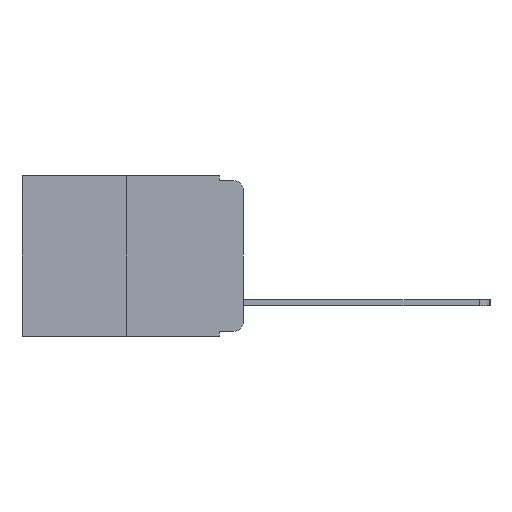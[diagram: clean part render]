
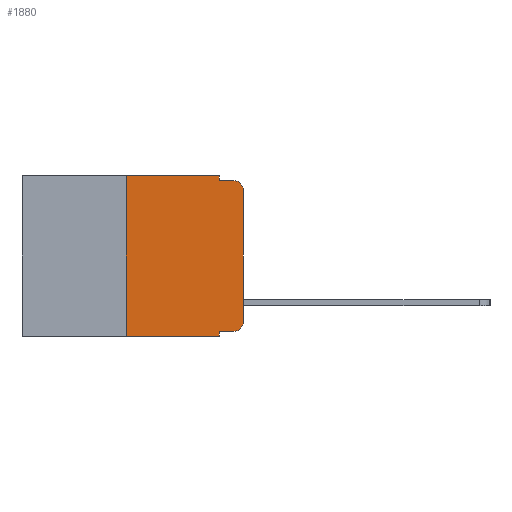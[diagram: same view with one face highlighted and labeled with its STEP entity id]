
A CAD part, left-side view. The second image highlights one B-rep face of the part: STEP entity #1880.
In plain terms, the highlighted planar face has unit normal (-1, 0, 0).
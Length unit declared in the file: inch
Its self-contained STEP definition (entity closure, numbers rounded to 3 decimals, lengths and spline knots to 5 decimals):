
#370 = LINE ( 'NONE', #4355, #4647 ) ;
#617 = EDGE_CURVE ( 'NONE', #16343, #2538, #10913, .T. ) ;
#1018 = LINE ( 'NONE', #10166, #6738 ) ;
#1031 = AXIS2_PLACEMENT_3D ( 'NONE', #2403, #11668, #3817 ) ;
#1208 = ORIENTED_EDGE ( 'NONE', *, *, #4333, .T. ) ;
#1236 = CIRCLE ( 'NONE', #12113, 0.02 ) ;
#1523 = ORIENTED_EDGE ( 'NONE', *, *, #617, .F. ) ;
#1568 = VERTEX_POINT ( 'NONE', #9383 ) ;
#1818 = VECTOR ( 'NONE', #5130, 39.37008 ) ;
#1880 = ADVANCED_FACE ( 'NONE', ( #2723 ), #7766, .F. ) ;
#2147 = VECTOR ( 'NONE', #4517, 39.37008 ) ;
#2393 = EDGE_CURVE ( 'NONE', #2538, #14943, #10297, .T. ) ;
#2403 = CARTESIAN_POINT ( 'NONE',  ( 0., 0.02, -0.03 ) ) ;
#2442 = VERTEX_POINT ( 'NONE', #16416 ) ;
#2538 = VERTEX_POINT ( 'NONE', #14724 ) ;
#2723 = FACE_OUTER_BOUND ( 'NONE', #16510, .T. ) ;
#2979 = VECTOR ( 'NONE', #11274, 39.37008 ) ;
#3442 = VECTOR ( 'NONE', #6699, 39.37008 ) ;
#3659 = DIRECTION ( 'NONE',  ( 0., -1., 0. ) ) ;
#3817 = DIRECTION ( 'NONE',  ( 0., 0., -1. ) ) ;
#4295 = EDGE_CURVE ( 'NONE', #6112, #16343, #1018, .T. ) ;
#4328 = EDGE_CURVE ( 'NONE', #10841, #12008, #16121, .T. ) ;
#4333 = EDGE_CURVE ( 'NONE', #10841, #8806, #5874, .T. ) ;
#4355 = CARTESIAN_POINT ( 'NONE',  ( 0., 0., 0. ) ) ;
#4384 = EDGE_CURVE ( 'NONE', #8806, #1568, #1236, .T. ) ;
#4517 = DIRECTION ( 'NONE',  ( 0., 0., -1. ) ) ;
#4647 = VECTOR ( 'NONE', #13317, 39.37008 ) ;
#5130 = DIRECTION ( 'NONE',  ( 0., 0., -1. ) ) ;
#5449 = VECTOR ( 'NONE', #12641, 39.37008 ) ;
#5874 = LINE ( 'NONE', #6305, #5449 ) ;
#5916 = EDGE_CURVE ( 'NONE', #6112, #12008, #16429, .T. ) ;
#6112 = VERTEX_POINT ( 'NONE', #13049 ) ;
#6175 = DIRECTION ( 'NONE',  ( 0., 0., -1. ) ) ;
#6223 = ORIENTED_EDGE ( 'NONE', *, *, #4328, .F. ) ;
#6305 = CARTESIAN_POINT ( 'NONE',  ( 0., 0.051, -0.333 ) ) ;
#6534 = ORIENTED_EDGE ( 'NONE', *, *, #2393, .F. ) ;
#6561 = VECTOR ( 'NONE', #3659, 39.37008 ) ;
#6634 = ORIENTED_EDGE ( 'NONE', *, *, #4295, .F. ) ;
#6699 = DIRECTION ( 'NONE',  ( 0., -1., 0. ) ) ;
#6738 = VECTOR ( 'NONE', #7012, 39.37008 ) ;
#6962 = ORIENTED_EDGE ( 'NONE', *, *, #7209, .T. ) ;
#6968 = DIRECTION ( 'NONE',  ( 1., 0., 0. ) ) ;
#6991 = LINE ( 'NONE', #11522, #6561 ) ;
#7012 = DIRECTION ( 'NONE',  ( 0., 0., 1. ) ) ;
#7209 = EDGE_CURVE ( 'NONE', #1568, #11190, #370, .T. ) ;
#7386 = DIRECTION ( 'NONE',  ( -1., 0., 0. ) ) ;
#7482 = CARTESIAN_POINT ( 'NONE',  ( 0., 0.473, -0.343 ) ) ;
#7766 = PLANE ( 'NONE',  #9470 ) ;
#8436 = CARTESIAN_POINT ( 'NONE',  ( 0., 0.051, -0.333 ) ) ;
#8806 = VERTEX_POINT ( 'NONE', #11986 ) ;
#8967 = ORIENTED_EDGE ( 'NONE', *, *, #5916, .T. ) ;
#8991 = CARTESIAN_POINT ( 'NONE',  ( 0., 0., -0.03 ) ) ;
#9383 = CARTESIAN_POINT ( 'NONE',  ( 0., 0., -0.313 ) ) ;
#9470 = AXIS2_PLACEMENT_3D ( 'NONE', #13332, #6968, #6175 ) ;
#9512 = ORIENTED_EDGE ( 'NONE', *, *, #10550, .T. ) ;
#9528 = CARTESIAN_POINT ( 'NONE',  ( 0., 0.473, 0. ) ) ;
#10166 = CARTESIAN_POINT ( 'NONE',  ( 0., 0.25, 0. ) ) ;
#10297 = LINE ( 'NONE', #16686, #1818 ) ;
#10337 = CARTESIAN_POINT ( 'NONE',  ( 0., 0.051, 0. ) ) ;
#10550 = EDGE_CURVE ( 'NONE', #11190, #2442, #11759, .T. ) ;
#10739 = CARTESIAN_POINT ( 'NONE',  ( 0., 0.25, 0. ) ) ;
#10841 = VERTEX_POINT ( 'NONE', #8436 ) ;
#10913 = LINE ( 'NONE', #9528, #3442 ) ;
#11190 = VERTEX_POINT ( 'NONE', #8991 ) ;
#11260 = ORIENTED_EDGE ( 'NONE', *, *, #11552, .F. ) ;
#11274 = DIRECTION ( 'NONE',  ( 0., -1., 0. ) ) ;
#11522 = CARTESIAN_POINT ( 'NONE',  ( 0., 0.051, -0.01 ) ) ;
#11552 = EDGE_CURVE ( 'NONE', #14943, #2442, #6991, .T. ) ;
#11668 = DIRECTION ( 'NONE',  ( -1., 0., 0. ) ) ;
#11723 = ORIENTED_EDGE ( 'NONE', *, *, #4384, .T. ) ;
#11759 = CIRCLE ( 'NONE', #1031, 0.02 ) ;
#11986 = CARTESIAN_POINT ( 'NONE',  ( 0., 0.02, -0.333 ) ) ;
#12008 = VERTEX_POINT ( 'NONE', #16639 ) ;
#12113 = AXIS2_PLACEMENT_3D ( 'NONE', #16451, #7386, #13482 ) ;
#12641 = DIRECTION ( 'NONE',  ( 0., -1., 0. ) ) ;
#13049 = CARTESIAN_POINT ( 'NONE',  ( 0., 0.25, -0.343 ) ) ;
#13317 = DIRECTION ( 'NONE',  ( 0., 0., 1. ) ) ;
#13332 = CARTESIAN_POINT ( 'NONE',  ( 0., 0.473, 0. ) ) ;
#13445 = CARTESIAN_POINT ( 'NONE',  ( 0., 0.051, -0.01 ) ) ;
#13482 = DIRECTION ( 'NONE',  ( 0., 0., -1. ) ) ;
#14724 = CARTESIAN_POINT ( 'NONE',  ( 0., 0.051, 0. ) ) ;
#14943 = VERTEX_POINT ( 'NONE', #13445 ) ;
#16121 = LINE ( 'NONE', #10337, #2147 ) ;
#16343 = VERTEX_POINT ( 'NONE', #10739 ) ;
#16416 = CARTESIAN_POINT ( 'NONE',  ( 0., 0.02, -0.01 ) ) ;
#16429 = LINE ( 'NONE', #7482, #2979 ) ;
#16451 = CARTESIAN_POINT ( 'NONE',  ( 0., 0.02, -0.313 ) ) ;
#16510 = EDGE_LOOP ( 'NONE', ( #6962, #9512, #11260, #6534, #1523, #6634, #8967, #6223, #1208, #11723 ) ) ;
#16639 = CARTESIAN_POINT ( 'NONE',  ( 0., 0.051, -0.343 ) ) ;
#16686 = CARTESIAN_POINT ( 'NONE',  ( 0., 0.051, 0. ) ) ;
